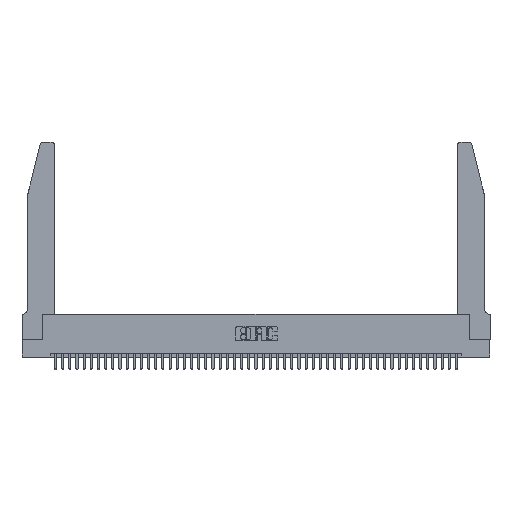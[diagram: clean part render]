
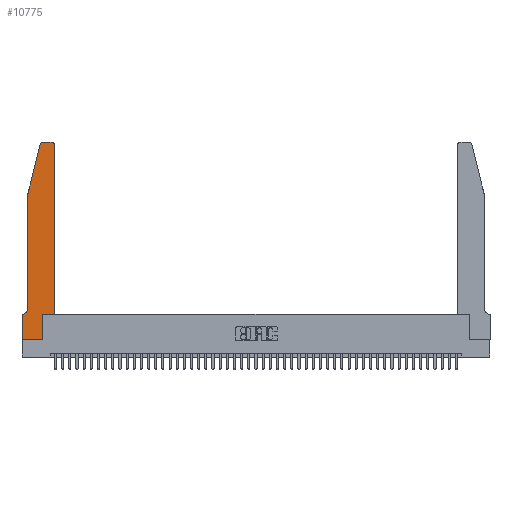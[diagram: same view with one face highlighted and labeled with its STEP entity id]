
A CAD part, top view. The second image highlights one B-rep face of the part: STEP entity #10775.
In plain terms, the highlighted planar face has unit normal (0, 0, 1).
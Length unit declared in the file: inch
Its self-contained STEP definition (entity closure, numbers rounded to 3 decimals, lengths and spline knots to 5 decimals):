
#9 = PLANE ( 'NONE',  #45324 ) ;
#68 = CARTESIAN_POINT ( 'NONE',  ( 0.25487, 2.72718, 0.37 ) ) ;
#1129 = LINE ( 'NONE', #26485, #46535 ) ;
#1528 = CARTESIAN_POINT ( 'NONE',  ( 0.2865, 0.35, 0.37 ) ) ;
#2419 = EDGE_CURVE ( 'NONE', #3314, #45678, #38023, .T. ) ;
#2613 = EDGE_CURVE ( 'NONE', #33160, #26165, #14506, .T. ) ;
#3090 = ORIENTED_EDGE ( 'NONE', *, *, #10563, .T. ) ;
#3314 = VERTEX_POINT ( 'NONE', #14519 ) ;
#3711 = DIRECTION ( 'NONE',  ( 0., 0., 1. ) ) ;
#3970 = AXIS2_PLACEMENT_3D ( 'NONE', #28558, #6497, #32268 ) ;
#5170 = ORIENTED_EDGE ( 'NONE', *, *, #21611, .T. ) ;
#5344 = VERTEX_POINT ( 'NONE', #18988 ) ;
#6463 = CIRCLE ( 'NONE', #3970, 0.07 ) ;
#6497 = DIRECTION ( 'NONE',  ( 0., 0., -1. ) ) ;
#7513 = CARTESIAN_POINT ( 'NONE',  ( 0.0755, 0.42, 0.37 ) ) ;
#8245 = VECTOR ( 'NONE', #25182, 39.37008 ) ;
#8267 = CARTESIAN_POINT ( 'NONE',  ( 0.2865, 0., 0.37 ) ) ;
#9009 = CARTESIAN_POINT ( 'NONE',  ( 0.4205, 2.72, 0.37 ) ) ;
#10040 = CARTESIAN_POINT ( 'NONE',  ( 0., 0., 0.37 ) ) ;
#10563 = EDGE_CURVE ( 'NONE', #46928, #3314, #44974, .T. ) ;
#10762 = DIRECTION ( 'NONE',  ( 0., 0., 1. ) ) ;
#10775 = ADVANCED_FACE ( 'NONE', ( #36971 ), #9, .T. ) ;
#12087 = CARTESIAN_POINT ( 'NONE',  ( 0.2865, 0.35, 0.37 ) ) ;
#12123 = CARTESIAN_POINT ( 'NONE',  ( 0., 0., 0.37 ) ) ;
#12651 = CARTESIAN_POINT ( 'NONE',  ( 0.0755, 2., 0.37 ) ) ;
#12730 = DIRECTION ( 'NONE',  ( 1., 0., 0. ) ) ;
#13747 = DIRECTION ( 'NONE',  ( 1., 0., 0. ) ) ;
#14098 = AXIS2_PLACEMENT_3D ( 'NONE', #9009, #34758, #12730 ) ;
#14506 = LINE ( 'NONE', #10040, #39202 ) ;
#14519 = CARTESIAN_POINT ( 'NONE',  ( 0.0755, 2., 0.37 ) ) ;
#15644 = AXIS2_PLACEMENT_3D ( 'NONE', #32800, #10762, #36511 ) ;
#15697 = VECTOR ( 'NONE', #28325, 39.37008 ) ;
#17013 = CIRCLE ( 'NONE', #14098, 0.03 ) ;
#18988 = CARTESIAN_POINT ( 'NONE',  ( 0.4505, 2.72, 0.37 ) ) ;
#20458 = CARTESIAN_POINT ( 'NONE',  ( 0.0055, 0.35, 0.37 ) ) ;
#20823 = VERTEX_POINT ( 'NONE', #29823 ) ;
#21484 = CARTESIAN_POINT ( 'NONE',  ( 0.4505, 0.35, 0.37 ) ) ;
#21611 = EDGE_CURVE ( 'NONE', #26165, #29131, #35139, .T. ) ;
#21621 = CARTESIAN_POINT ( 'NONE',  ( 0.4505, 0.35, 0.37 ) ) ;
#21660 = VECTOR ( 'NONE', #37160, 39.37008 ) ;
#21712 = EDGE_CURVE ( 'NONE', #25507, #20823, #32837, .T. ) ;
#22044 = CARTESIAN_POINT ( 'NONE',  ( 0., 0.35, 0.37 ) ) ;
#22555 = VERTEX_POINT ( 'NONE', #24516 ) ;
#22806 = EDGE_LOOP ( 'NONE', ( #30216, #35369, #3090, #31665, #41317, #32360, #34532, #27447, #5170, #32632, #35846, #32809 ) ) ;
#23048 = VERTEX_POINT ( 'NONE', #20458 ) ;
#23879 = CIRCLE ( 'NONE', #15644, 0.03 ) ;
#24516 = CARTESIAN_POINT ( 'NONE',  ( 0., 0.35, 0.37 ) ) ;
#24956 = EDGE_CURVE ( 'NONE', #5344, #25507, #17013, .T. ) ;
#25171 = VECTOR ( 'NONE', #41820, 39.37008 ) ;
#25182 = DIRECTION ( 'NONE',  ( 1., 0., 0. ) ) ;
#25257 = EDGE_CURVE ( 'NONE', #20823, #46928, #23879, .T. ) ;
#25342 = VECTOR ( 'NONE', #45136, 39.37008 ) ;
#25507 = VERTEX_POINT ( 'NONE', #41765 ) ;
#25828 = EDGE_CURVE ( 'NONE', #29131, #38245, #37630, .T. ) ;
#26165 = VERTEX_POINT ( 'NONE', #8267 ) ;
#26485 = CARTESIAN_POINT ( 'NONE',  ( 0., 0., 0.37 ) ) ;
#27052 = CARTESIAN_POINT ( 'NONE',  ( 0.4505, 0.35, 0.37 ) ) ;
#27447 = ORIENTED_EDGE ( 'NONE', *, *, #2613, .T. ) ;
#27478 = CARTESIAN_POINT ( 'NONE',  ( 0.2605, 2.75, 0.37 ) ) ;
#28325 = DIRECTION ( 'NONE',  ( -0.239, -0.971, 0. ) ) ;
#28558 = CARTESIAN_POINT ( 'NONE',  ( 0.0055, 0.42, 0.37 ) ) ;
#29131 = VERTEX_POINT ( 'NONE', #1528 ) ;
#29435 = DIRECTION ( 'NONE',  ( 1., 0., 0. ) ) ;
#29823 = CARTESIAN_POINT ( 'NONE',  ( 0.284, 2.75, 0.37 ) ) ;
#30216 = ORIENTED_EDGE ( 'NONE', *, *, #21712, .T. ) ;
#30836 = EDGE_CURVE ( 'NONE', #23048, #22555, #41198, .T. ) ;
#31197 = DIRECTION ( 'NONE',  ( -1., 0., 0. ) ) ;
#31665 = ORIENTED_EDGE ( 'NONE', *, *, #2419, .T. ) ;
#32268 = DIRECTION ( 'NONE',  ( -1., 0., 0. ) ) ;
#32360 = ORIENTED_EDGE ( 'NONE', *, *, #30836, .T. ) ;
#32632 = ORIENTED_EDGE ( 'NONE', *, *, #25828, .T. ) ;
#32800 = CARTESIAN_POINT ( 'NONE',  ( 0.284, 2.72, 0.37 ) ) ;
#32809 = ORIENTED_EDGE ( 'NONE', *, *, #24956, .T. ) ;
#32837 = LINE ( 'NONE', #27478, #40249 ) ;
#33160 = VERTEX_POINT ( 'NONE', #12123 ) ;
#33455 = CARTESIAN_POINT ( 'NONE',  ( 0.0755, 0.35, 0.37 ) ) ;
#34056 = DIRECTION ( 'NONE',  ( 0., -1., 0. ) ) ;
#34532 = ORIENTED_EDGE ( 'NONE', *, *, #46414, .T. ) ;
#34758 = DIRECTION ( 'NONE',  ( 0., 0., 1. ) ) ;
#34980 = LINE ( 'NONE', #27052, #25171 ) ;
#35118 = EDGE_CURVE ( 'NONE', #38245, #5344, #34980, .T. ) ;
#35139 = LINE ( 'NONE', #12087, #25342 ) ;
#35369 = ORIENTED_EDGE ( 'NONE', *, *, #25257, .T. ) ;
#35846 = ORIENTED_EDGE ( 'NONE', *, *, #35118, .T. ) ;
#36511 = DIRECTION ( 'NONE',  ( 1., 0., 0. ) ) ;
#36889 = VECTOR ( 'NONE', #45702, 39.37008 ) ;
#36971 = FACE_OUTER_BOUND ( 'NONE', #22806, .T. ) ;
#37160 = DIRECTION ( 'NONE',  ( -1., 0., 0. ) ) ;
#37630 = LINE ( 'NONE', #21484, #8245 ) ;
#38023 = LINE ( 'NONE', #12651, #36889 ) ;
#38245 = VERTEX_POINT ( 'NONE', #21621 ) ;
#39202 = VECTOR ( 'NONE', #13747, 39.37008 ) ;
#40249 = VECTOR ( 'NONE', #31197, 39.37008 ) ;
#41198 = LINE ( 'NONE', #33455, #21660 ) ;
#41317 = ORIENTED_EDGE ( 'NONE', *, *, #43186, .T. ) ;
#41765 = CARTESIAN_POINT ( 'NONE',  ( 0.4205, 2.75, 0.37 ) ) ;
#41820 = DIRECTION ( 'NONE',  ( 0., 1., 0. ) ) ;
#42921 = CARTESIAN_POINT ( 'NONE',  ( 0.0755, 2., 0.37 ) ) ;
#43186 = EDGE_CURVE ( 'NONE', #45678, #23048, #6463, .T. ) ;
#44974 = LINE ( 'NONE', #42921, #15697 ) ;
#45136 = DIRECTION ( 'NONE',  ( 0., 1., 0. ) ) ;
#45324 = AXIS2_PLACEMENT_3D ( 'NONE', #22044, #3711, #29435 ) ;
#45678 = VERTEX_POINT ( 'NONE', #7513 ) ;
#45702 = DIRECTION ( 'NONE',  ( 0., -1., 0. ) ) ;
#46414 = EDGE_CURVE ( 'NONE', #22555, #33160, #1129, .T. ) ;
#46535 = VECTOR ( 'NONE', #34056, 39.37008 ) ;
#46928 = VERTEX_POINT ( 'NONE', #68 ) ;
